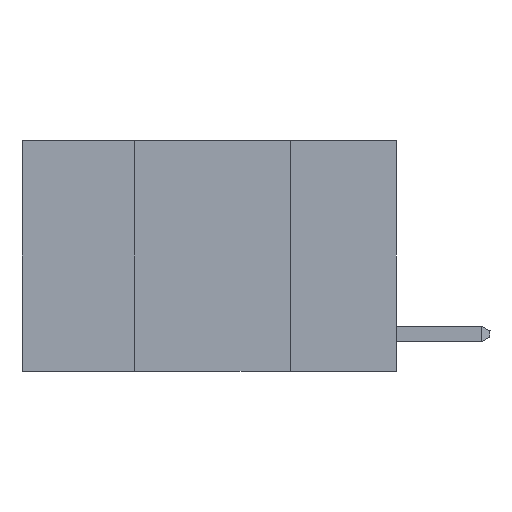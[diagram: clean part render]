
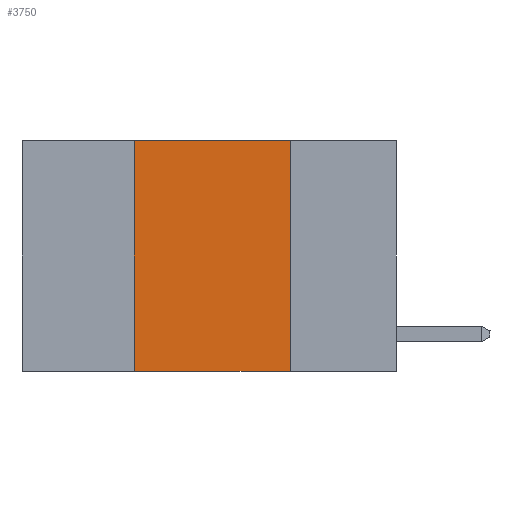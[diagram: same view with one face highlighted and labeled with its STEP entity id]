
A CAD part, left-side view. The second image highlights one B-rep face of the part: STEP entity #3750.
In plain terms, the highlighted planar face has unit normal (-1, 0, 0).
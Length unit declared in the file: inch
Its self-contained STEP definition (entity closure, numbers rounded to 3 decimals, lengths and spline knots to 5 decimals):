
#640 = DIRECTION ( 'NONE',  ( 0., -1., 0. ) ) ;
#1189 = VECTOR ( 'NONE', #26477, 39.37008 ) ;
#1494 = VERTEX_POINT ( 'NONE', #17890 ) ;
#1971 = AXIS2_PLACEMENT_3D ( 'NONE', #12036, #26575, #14135 ) ;
#2481 = DIRECTION ( 'NONE',  ( 0., -1., 0. ) ) ;
#2790 = EDGE_CURVE ( 'NONE', #18616, #1494, #24670, .T. ) ;
#3750 = ADVANCED_FACE ( 'NONE', ( #6568 ), #24486, .F. ) ;
#3840 = EDGE_LOOP ( 'NONE', ( #12307, #24033, #8109, #19790 ) ) ;
#6568 = FACE_OUTER_BOUND ( 'NONE', #3840, .T. ) ;
#6738 = EDGE_CURVE ( 'NONE', #19565, #26760, #13881, .T. ) ;
#8109 = ORIENTED_EDGE ( 'NONE', *, *, #8139, .F. ) ;
#8139 = EDGE_CURVE ( 'NONE', #19565, #18616, #17732, .T. ) ;
#8844 = VECTOR ( 'NONE', #14925, 39.37008 ) ;
#12036 = CARTESIAN_POINT ( 'NONE',  ( 0., 0.6, 0. ) ) ;
#12307 = ORIENTED_EDGE ( 'NONE', *, *, #16448, .F. ) ;
#12837 = CARTESIAN_POINT ( 'NONE',  ( 0., 0.17, 0. ) ) ;
#13881 = LINE ( 'NONE', #15169, #19390 ) ;
#14135 = DIRECTION ( 'NONE',  ( 0., 0., -1. ) ) ;
#14925 = DIRECTION ( 'NONE',  ( 0., 0., -1. ) ) ;
#15169 = CARTESIAN_POINT ( 'NONE',  ( 0., 0.6, -0.37 ) ) ;
#16448 = EDGE_CURVE ( 'NONE', #1494, #26760, #19864, .T. ) ;
#17732 = LINE ( 'NONE', #26392, #1189 ) ;
#17890 = CARTESIAN_POINT ( 'NONE',  ( 0., 0.17, 0. ) ) ;
#18616 = VERTEX_POINT ( 'NONE', #19881 ) ;
#19390 = VECTOR ( 'NONE', #640, 39.37008 ) ;
#19565 = VERTEX_POINT ( 'NONE', #22750 ) ;
#19790 = ORIENTED_EDGE ( 'NONE', *, *, #6738, .T. ) ;
#19864 = LINE ( 'NONE', #12837, #8844 ) ;
#19881 = CARTESIAN_POINT ( 'NONE',  ( 0., 0.42, 0. ) ) ;
#22750 = CARTESIAN_POINT ( 'NONE',  ( 0., 0.42, -0.37 ) ) ;
#23381 = CARTESIAN_POINT ( 'NONE',  ( 0., 0.17, -0.37 ) ) ;
#24028 = VECTOR ( 'NONE', #2481, 39.37008 ) ;
#24033 = ORIENTED_EDGE ( 'NONE', *, *, #2790, .F. ) ;
#24486 = PLANE ( 'NONE',  #1971 ) ;
#24670 = LINE ( 'NONE', #25255, #24028 ) ;
#25255 = CARTESIAN_POINT ( 'NONE',  ( 0., 0.6, 0. ) ) ;
#26392 = CARTESIAN_POINT ( 'NONE',  ( 0., 0.42, 0. ) ) ;
#26477 = DIRECTION ( 'NONE',  ( 0., 0., 1. ) ) ;
#26575 = DIRECTION ( 'NONE',  ( 1., 0., 0. ) ) ;
#26760 = VERTEX_POINT ( 'NONE', #23381 ) ;
